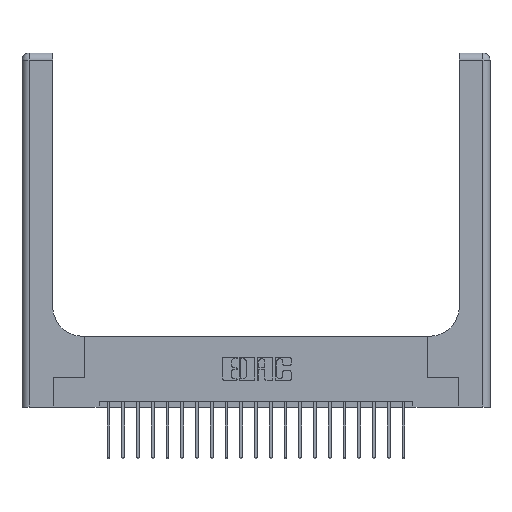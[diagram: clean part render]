
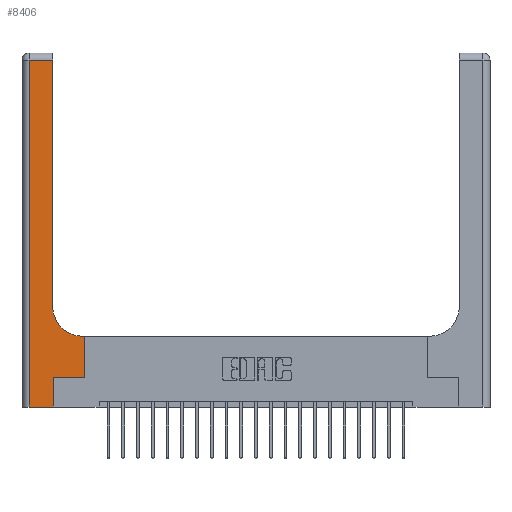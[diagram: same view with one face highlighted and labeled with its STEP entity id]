
A CAD part, top view. The second image highlights one B-rep face of the part: STEP entity #8406.
In plain terms, the highlighted planar face has unit normal (0, 0, 1).
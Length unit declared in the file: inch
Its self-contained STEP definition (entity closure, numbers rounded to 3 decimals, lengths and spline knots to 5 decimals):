
#94 = EDGE_CURVE ( 'NONE', #21184, #15094, #1519, .T. ) ;
#113 = LINE ( 'NONE', #10104, #3506 ) ;
#240 = CARTESIAN_POINT ( 'NONE',  ( 0.265, 0.25, 0.37 ) ) ;
#1027 = CARTESIAN_POINT ( 'NONE',  ( 0.06, 2.94, 0.37 ) ) ;
#1159 = LINE ( 'NONE', #13463, #9062 ) ;
#1519 = LINE ( 'NONE', #21306, #2788 ) ;
#2595 = CARTESIAN_POINT ( 'NONE',  ( 0.26, 0.85, 0.37 ) ) ;
#2663 = CARTESIAN_POINT ( 'NONE',  ( 0., 0., 0.37 ) ) ;
#2788 = VECTOR ( 'NONE', #2838, 39.37008 ) ;
#2838 = DIRECTION ( 'NONE',  ( 0., 1., 0. ) ) ;
#3268 = VECTOR ( 'NONE', #10165, 39.37008 ) ;
#3506 = VECTOR ( 'NONE', #12007, 39.37008 ) ;
#3554 = LINE ( 'NONE', #11494, #3268 ) ;
#3849 = DIRECTION ( 'NONE',  ( 0., 0., -1. ) ) ;
#3992 = VECTOR ( 'NONE', #16031, 39.37008 ) ;
#4116 = VERTEX_POINT ( 'NONE', #1027 ) ;
#4123 = CARTESIAN_POINT ( 'NONE',  ( 0.06, 0., 0.37 ) ) ;
#4326 = AXIS2_PLACEMENT_3D ( 'NONE', #15748, #3849, #7267 ) ;
#4930 = LINE ( 'NONE', #240, #15957 ) ;
#5795 = LINE ( 'NONE', #10036, #17058 ) ;
#6339 = VERTEX_POINT ( 'NONE', #17964 ) ;
#6765 = VECTOR ( 'NONE', #13054, 39.37008 ) ;
#6870 = DIRECTION ( 'NONE',  ( 1., 0., 0. ) ) ;
#7267 = DIRECTION ( 'NONE',  ( -1., 0., 0. ) ) ;
#7518 = VERTEX_POINT ( 'NONE', #12160 ) ;
#7687 = EDGE_CURVE ( 'NONE', #7518, #15864, #11208, .T. ) ;
#8245 = EDGE_LOOP ( 'NONE', ( #12367, #15078, #21543, #8652, #15237, #19996, #16496, #9694, #16996 ) ) ;
#8406 = ADVANCED_FACE ( 'NONE', ( #19841 ), #17276, .F. ) ;
#8652 = ORIENTED_EDGE ( 'NONE', *, *, #10042, .T. ) ;
#9062 = VECTOR ( 'NONE', #15448, 39.37008 ) ;
#9090 = CARTESIAN_POINT ( 'NONE',  ( 0.528, 0.6, 0.37 ) ) ;
#9113 = EDGE_CURVE ( 'NONE', #6339, #4116, #113, .T. ) ;
#9115 = EDGE_CURVE ( 'NONE', #15094, #13080, #1159, .T. ) ;
#9694 = ORIENTED_EDGE ( 'NONE', *, *, #9115, .T. ) ;
#10036 = CARTESIAN_POINT ( 'NONE',  ( 0.26, 3., 0.37 ) ) ;
#10042 = EDGE_CURVE ( 'NONE', #12768, #7518, #13455, .T. ) ;
#10104 = CARTESIAN_POINT ( 'NONE',  ( 0., 2.94, 0.37 ) ) ;
#10110 = DIRECTION ( 'NONE',  ( 0., 1., 0. ) ) ;
#10139 = AXIS2_PLACEMENT_3D ( 'NONE', #15720, #12492, #19312 ) ;
#10165 = DIRECTION ( 'NONE',  ( 0., -1., 0. ) ) ;
#10301 = CIRCLE ( 'NONE', #10139, 0.25 ) ;
#10737 = EDGE_CURVE ( 'NONE', #13080, #17779, #10301, .T. ) ;
#11208 = LINE ( 'NONE', #12508, #6765 ) ;
#11494 = CARTESIAN_POINT ( 'NONE',  ( 0.06, 3., 0.37 ) ) ;
#12007 = DIRECTION ( 'NONE',  ( -1., 0., 0. ) ) ;
#12160 = CARTESIAN_POINT ( 'NONE',  ( 0.265, 0., 0.37 ) ) ;
#12367 = ORIENTED_EDGE ( 'NONE', *, *, #17916, .T. ) ;
#12492 = DIRECTION ( 'NONE',  ( 0., 0., -1. ) ) ;
#12508 = CARTESIAN_POINT ( 'NONE',  ( 0.265, 0., 0.37 ) ) ;
#12768 = VERTEX_POINT ( 'NONE', #4123 ) ;
#13054 = DIRECTION ( 'NONE',  ( 0., 1., 0. ) ) ;
#13080 = VERTEX_POINT ( 'NONE', #19518 ) ;
#13455 = LINE ( 'NONE', #2663, #3992 ) ;
#13463 = CARTESIAN_POINT ( 'NONE',  ( 0.26, 0.6, 0.37 ) ) ;
#15078 = ORIENTED_EDGE ( 'NONE', *, *, #9113, .T. ) ;
#15094 = VERTEX_POINT ( 'NONE', #9090 ) ;
#15237 = ORIENTED_EDGE ( 'NONE', *, *, #7687, .T. ) ;
#15448 = DIRECTION ( 'NONE',  ( -1., 0., 0. ) ) ;
#15720 = CARTESIAN_POINT ( 'NONE',  ( 0.51, 0.85, 0.37 ) ) ;
#15748 = CARTESIAN_POINT ( 'NONE',  ( 0., 3., 0.37 ) ) ;
#15864 = VERTEX_POINT ( 'NONE', #17357 ) ;
#15957 = VECTOR ( 'NONE', #6870, 39.37008 ) ;
#16031 = DIRECTION ( 'NONE',  ( 1., 0., 0. ) ) ;
#16496 = ORIENTED_EDGE ( 'NONE', *, *, #94, .T. ) ;
#16996 = ORIENTED_EDGE ( 'NONE', *, *, #10737, .T. ) ;
#17058 = VECTOR ( 'NONE', #10110, 39.37008 ) ;
#17276 = PLANE ( 'NONE',  #4326 ) ;
#17357 = CARTESIAN_POINT ( 'NONE',  ( 0.265, 0.25, 0.37 ) ) ;
#17779 = VERTEX_POINT ( 'NONE', #2595 ) ;
#17916 = EDGE_CURVE ( 'NONE', #17779, #6339, #5795, .T. ) ;
#17964 = CARTESIAN_POINT ( 'NONE',  ( 0.26, 2.94, 0.37 ) ) ;
#18443 = CARTESIAN_POINT ( 'NONE',  ( 0.528, 0.25, 0.37 ) ) ;
#19240 = EDGE_CURVE ( 'NONE', #15864, #21184, #4930, .T. ) ;
#19312 = DIRECTION ( 'NONE',  ( 1., 0., 0. ) ) ;
#19518 = CARTESIAN_POINT ( 'NONE',  ( 0.51, 0.6, 0.37 ) ) ;
#19841 = FACE_OUTER_BOUND ( 'NONE', #8245, .T. ) ;
#19996 = ORIENTED_EDGE ( 'NONE', *, *, #19240, .T. ) ;
#21068 = EDGE_CURVE ( 'NONE', #4116, #12768, #3554, .T. ) ;
#21184 = VERTEX_POINT ( 'NONE', #18443 ) ;
#21306 = CARTESIAN_POINT ( 'NONE',  ( 0.528, 0.25, 0.37 ) ) ;
#21543 = ORIENTED_EDGE ( 'NONE', *, *, #21068, .T. ) ;
